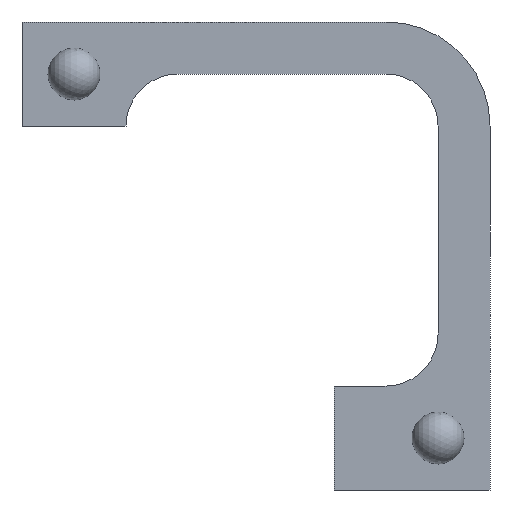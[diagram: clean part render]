
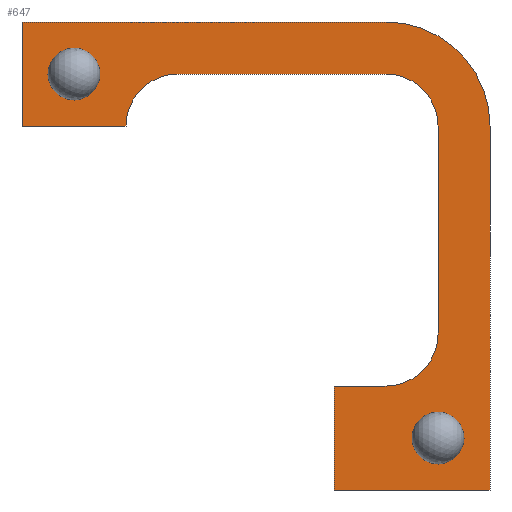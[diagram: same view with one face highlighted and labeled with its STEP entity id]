
A CAD part, left-side view. The second image highlights one B-rep face of the part: STEP entity #647.
In plain terms, the highlighted planar face has unit normal (-1, 0, 0).
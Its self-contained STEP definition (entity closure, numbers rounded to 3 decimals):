
#3 = CARTESIAN_POINT ( 'NONE',  ( 0., 5., 10. ) ) ;
#6 = AXIS2_PLACEMENT_3D ( 'NONE', #640, #358, #39 ) ;
#9 = VERTEX_POINT ( 'NONE', #413 ) ;
#10 = ORIENTED_EDGE ( 'NONE', *, *, #326, .T. ) ;
#12 = CIRCLE ( 'NONE', #50, 10. ) ;
#14 = DIRECTION ( 'NONE',  ( 0., 0., -1. ) ) ;
#16 = DIRECTION ( 'NONE',  ( 1., 0., 0. ) ) ;
#17 = ORIENTED_EDGE ( 'NONE', *, *, #346, .T. ) ;
#18 = EDGE_LOOP ( 'NONE', ( #438, #17 ) ) ;
#25 = CARTESIAN_POINT ( 'NONE',  ( 0., -25., -25. ) ) ;
#28 = VERTEX_POINT ( 'NONE', #392 ) ;
#30 = CARTESIAN_POINT ( 'NONE',  ( 0., 15., 15. ) ) ;
#32 = VECTOR ( 'NONE', #296, 1000. ) ;
#33 = CARTESIAN_POINT ( 'NONE',  ( 0., 0., -15. ) ) ;
#35 = ORIENTED_EDGE ( 'NONE', *, *, #112, .F. ) ;
#39 = DIRECTION ( 'NONE',  ( 0., 0., -1. ) ) ;
#43 = CARTESIAN_POINT ( 'NONE',  ( 0., 5., 15. ) ) ;
#50 = AXIS2_PLACEMENT_3D ( 'NONE', #76, #420, #132 ) ;
#51 = LINE ( 'NONE', #560, #32 ) ;
#53 = CARTESIAN_POINT ( 'NONE',  ( 0., 20., 20. ) ) ;
#56 = CARTESIAN_POINT ( 'NONE',  ( 0., -20., 10. ) ) ;
#63 = CIRCLE ( 'NONE', #67, 5. ) ;
#67 = AXIS2_PLACEMENT_3D ( 'NONE', #3, #505, #239 ) ;
#68 = VERTEX_POINT ( 'NONE', #600 ) ;
#76 = CARTESIAN_POINT ( 'NONE',  ( 0., -15., 10. ) ) ;
#111 = CARTESIAN_POINT ( 'NONE',  ( 0., 0., 20. ) ) ;
#112 = EDGE_CURVE ( 'NONE', #489, #125, #400, .T. ) ;
#113 = CARTESIAN_POINT ( 'NONE',  ( 0., 15., 12.5 ) ) ;
#125 = VERTEX_POINT ( 'NONE', #348 ) ;
#131 = CARTESIAN_POINT ( 'NONE',  ( 0., -20., -17.5 ) ) ;
#132 = DIRECTION ( 'NONE',  ( 0., 0., -1. ) ) ;
#135 = ORIENTED_EDGE ( 'NONE', *, *, #374, .T. ) ;
#137 = VERTEX_POINT ( 'NONE', #507 ) ;
#138 = VERTEX_POINT ( 'NONE', #257 ) ;
#150 = VERTEX_POINT ( 'NONE', #522 ) ;
#152 = VERTEX_POINT ( 'NONE', #113 ) ;
#153 = DIRECTION ( 'NONE',  ( 0., -1., 0. ) ) ;
#162 = DIRECTION ( 'NONE',  ( 0., 0., -1. ) ) ;
#171 = DIRECTION ( 'NONE',  ( 1., 0., 0. ) ) ;
#172 = EDGE_LOOP ( 'NONE', ( #471, #268, #230, #439, #523, #581, #652, #135, #187, #456, #488, #578, #35 ) ) ;
#175 = CARTESIAN_POINT ( 'NONE',  ( 0., -15., 10. ) ) ;
#176 = FACE_OUTER_BOUND ( 'NONE', #172, .T. ) ;
#184 = PLANE ( 'NONE',  #610 ) ;
#186 = DIRECTION ( 'NONE',  ( 1., 0., 0. ) ) ;
#187 = ORIENTED_EDGE ( 'NONE', *, *, #646, .F. ) ;
#189 = VERTEX_POINT ( 'NONE', #633 ) ;
#197 = FACE_BOUND ( 'NONE', #18, .T. ) ;
#198 = AXIS2_PLACEMENT_3D ( 'NONE', #30, #16, #14 ) ;
#202 = CIRCLE ( 'NONE', #220, 5. ) ;
#211 = AXIS2_PLACEMENT_3D ( 'NONE', #262, #260, #258 ) ;
#220 = AXIS2_PLACEMENT_3D ( 'NONE', #175, #171, #162 ) ;
#224 = VECTOR ( 'NONE', #366, 1000. ) ;
#229 = CARTESIAN_POINT ( 'NONE',  ( 0., 0., 0. ) ) ;
#230 = ORIENTED_EDGE ( 'NONE', *, *, #306, .F. ) ;
#232 = CARTESIAN_POINT ( 'NONE',  ( 0., -25., 0. ) ) ;
#233 = LINE ( 'NONE', #33, #224 ) ;
#237 = DIRECTION ( 'NONE',  ( 0., 0., -1. ) ) ;
#239 = DIRECTION ( 'NONE',  ( 0., 0., -1. ) ) ;
#240 = VERTEX_POINT ( 'NONE', #468 ) ;
#252 = CIRCLE ( 'NONE', #211, 2.5 ) ;
#255 = CARTESIAN_POINT ( 'NONE',  ( 0., -15., 15. ) ) ;
#257 = CARTESIAN_POINT ( 'NONE',  ( 0., 20., 10. ) ) ;
#258 = DIRECTION ( 'NONE',  ( 0., 0., -1. ) ) ;
#260 = DIRECTION ( 'NONE',  ( 1., 0., 0. ) ) ;
#262 = CARTESIAN_POINT ( 'NONE',  ( 0., -20., -20. ) ) ;
#264 = CIRCLE ( 'NONE', #198, 2.5 ) ;
#268 = ORIENTED_EDGE ( 'NONE', *, *, #532, .T. ) ;
#271 = LINE ( 'NONE', #111, #272 ) ;
#272 = VECTOR ( 'NONE', #153, 1000. ) ;
#273 = VECTOR ( 'NONE', #237, 1000. ) ;
#274 = EDGE_CURVE ( 'NONE', #460, #138, #309, .T. ) ;
#277 = EDGE_CURVE ( 'NONE', #28, #424, #323, .T. ) ;
#279 = LINE ( 'NONE', #232, #273 ) ;
#287 = DIRECTION ( 'NONE',  ( 0., 0., -1. ) ) ;
#295 = EDGE_CURVE ( 'NONE', #593, #489, #279, .T. ) ;
#296 = DIRECTION ( 'NONE',  ( 0., -1., 0. ) ) ;
#306 = EDGE_CURVE ( 'NONE', #460, #240, #271, .T. ) ;
#308 = VECTOR ( 'NONE', #497, 1000. ) ;
#309 = LINE ( 'NONE', #319, #308 ) ;
#319 = CARTESIAN_POINT ( 'NONE',  ( 0., 20., 0. ) ) ;
#323 = CIRCLE ( 'NONE', #429, 2.5 ) ;
#326 = EDGE_CURVE ( 'NONE', #152, #189, #264, .T. ) ;
#327 = VERTEX_POINT ( 'NONE', #43 ) ;
#332 = EDGE_CURVE ( 'NONE', #9, #150, #233, .T. ) ;
#340 = CARTESIAN_POINT ( 'NONE',  ( 0., 10., 15. ) ) ;
#346 = EDGE_CURVE ( 'NONE', #424, #28, #252, .T. ) ;
#348 = CARTESIAN_POINT ( 'NONE',  ( 0., -10., -25. ) ) ;
#358 = DIRECTION ( 'NONE',  ( 1., 0., 0. ) ) ;
#366 = DIRECTION ( 'NONE',  ( 0., 1., 0. ) ) ;
#374 = EDGE_CURVE ( 'NONE', #644, #457, #202, .T. ) ;
#376 = DIRECTION ( 'NONE',  ( 1., 0., 0. ) ) ;
#392 = CARTESIAN_POINT ( 'NONE',  ( 0., -20., -22.5 ) ) ;
#395 = VECTOR ( 'NONE', #609, 1000. ) ;
#398 = CARTESIAN_POINT ( 'NONE',  ( 0., -20., 15. ) ) ;
#400 = LINE ( 'NONE', #531, #395 ) ;
#413 = CARTESIAN_POINT ( 'NONE',  ( 0., -15., -15. ) ) ;
#420 = DIRECTION ( 'NONE',  ( -1., 0., 0. ) ) ;
#424 = VERTEX_POINT ( 'NONE', #131 ) ;
#429 = AXIS2_PLACEMENT_3D ( 'NONE', #538, #376, #478 ) ;
#438 = ORIENTED_EDGE ( 'NONE', *, *, #277, .T. ) ;
#439 = ORIENTED_EDGE ( 'NONE', *, *, #274, .T. ) ;
#452 = EDGE_LOOP ( 'NONE', ( #10, #566 ) ) ;
#455 = DIRECTION ( 'NONE',  ( 0., 0., 1. ) ) ;
#456 = ORIENTED_EDGE ( 'NONE', *, *, #625, .T. ) ;
#457 = VERTEX_POINT ( 'NONE', #56 ) ;
#458 = CARTESIAN_POINT ( 'NONE',  ( 0., 15., 15. ) ) ;
#460 = VERTEX_POINT ( 'NONE', #53 ) ;
#468 = CARTESIAN_POINT ( 'NONE',  ( 0., -15., 20. ) ) ;
#471 = ORIENTED_EDGE ( 'NONE', *, *, #295, .F. ) ;
#476 = DIRECTION ( 'NONE',  ( 0., 0., 1. ) ) ;
#478 = DIRECTION ( 'NONE',  ( 0., 0., -1. ) ) ;
#486 = EDGE_CURVE ( 'NONE', #68, #327, #63, .T. ) ;
#488 = ORIENTED_EDGE ( 'NONE', *, *, #332, .T. ) ;
#489 = VERTEX_POINT ( 'NONE', #25 ) ;
#494 = EDGE_CURVE ( 'NONE', #138, #68, #51, .T. ) ;
#497 = DIRECTION ( 'NONE',  ( 0., 0., -1. ) ) ;
#502 = DIRECTION ( 'NONE',  ( 0., 0., -1. ) ) ;
#505 = DIRECTION ( 'NONE',  ( 1., 0., 0. ) ) ;
#507 = CARTESIAN_POINT ( 'NONE',  ( 0., -20., -10. ) ) ;
#522 = CARTESIAN_POINT ( 'NONE',  ( 0., -10., -15. ) ) ;
#523 = ORIENTED_EDGE ( 'NONE', *, *, #494, .T. ) ;
#524 = CIRCLE ( 'NONE', #617, 2.5 ) ;
#531 = CARTESIAN_POINT ( 'NONE',  ( 0., 0., -25. ) ) ;
#532 = EDGE_CURVE ( 'NONE', #593, #240, #12, .T. ) ;
#533 = VECTOR ( 'NONE', #607, 1000. ) ;
#538 = CARTESIAN_POINT ( 'NONE',  ( 0., -20., -20. ) ) ;
#550 = LINE ( 'NONE', #340, #533 ) ;
#551 = VECTOR ( 'NONE', #455, 1000. ) ;
#552 = DIRECTION ( 'NONE',  ( 1., 0., 0. ) ) ;
#560 = CARTESIAN_POINT ( 'NONE',  ( 0., 0., 10. ) ) ;
#561 = LINE ( 'NONE', #398, #551 ) ;
#562 = FACE_BOUND ( 'NONE', #452, .T. ) ;
#566 = ORIENTED_EDGE ( 'NONE', *, *, #659, .T. ) ;
#574 = VECTOR ( 'NONE', #476, 1000. ) ;
#576 = CARTESIAN_POINT ( 'NONE',  ( 0., -25., 10. ) ) ;
#578 = ORIENTED_EDGE ( 'NONE', *, *, #611, .F. ) ;
#581 = ORIENTED_EDGE ( 'NONE', *, *, #486, .T. ) ;
#585 = CIRCLE ( 'NONE', #6, 5. ) ;
#593 = VERTEX_POINT ( 'NONE', #576 ) ;
#600 = CARTESIAN_POINT ( 'NONE',  ( 0., 10., 10. ) ) ;
#607 = DIRECTION ( 'NONE',  ( 0., 1., 0. ) ) ;
#609 = DIRECTION ( 'NONE',  ( 0., 1., 0. ) ) ;
#610 = AXIS2_PLACEMENT_3D ( 'NONE', #229, #552, #287 ) ;
#611 = EDGE_CURVE ( 'NONE', #125, #150, #613, .T. ) ;
#613 = LINE ( 'NONE', #631, #574 ) ;
#617 = AXIS2_PLACEMENT_3D ( 'NONE', #458, #186, #502 ) ;
#625 = EDGE_CURVE ( 'NONE', #137, #9, #585, .T. ) ;
#631 = CARTESIAN_POINT ( 'NONE',  ( 0., -10., 0. ) ) ;
#633 = CARTESIAN_POINT ( 'NONE',  ( 0., 15., 17.5 ) ) ;
#640 = CARTESIAN_POINT ( 'NONE',  ( 0., -15., -10. ) ) ;
#644 = VERTEX_POINT ( 'NONE', #255 ) ;
#646 = EDGE_CURVE ( 'NONE', #137, #457, #561, .T. ) ;
#647 = ADVANCED_FACE ( 'NONE', ( #197, #562, #176 ), #184, .F. ) ;
#652 = ORIENTED_EDGE ( 'NONE', *, *, #653, .F. ) ;
#653 = EDGE_CURVE ( 'NONE', #644, #327, #550, .T. ) ;
#659 = EDGE_CURVE ( 'NONE', #189, #152, #524, .T. ) ;
